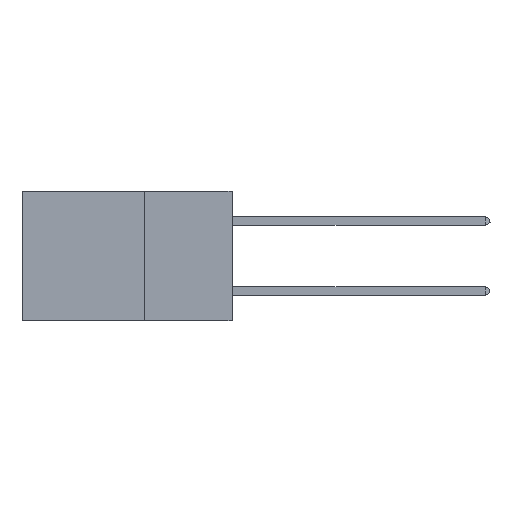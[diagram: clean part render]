
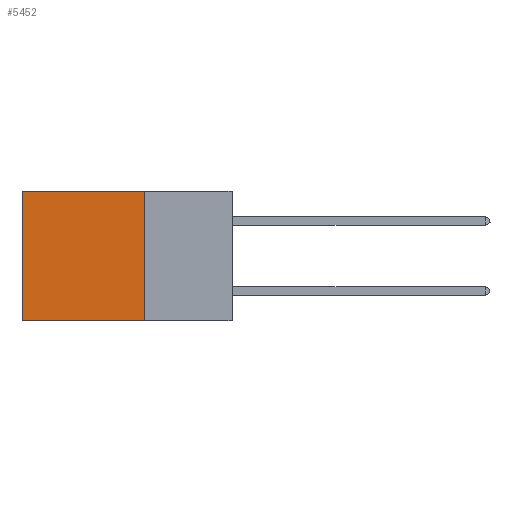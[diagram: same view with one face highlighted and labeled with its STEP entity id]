
A CAD part, left-side view. The second image highlights one B-rep face of the part: STEP entity #5452.
In plain terms, the highlighted planar face has unit normal (-1, 0, 0).
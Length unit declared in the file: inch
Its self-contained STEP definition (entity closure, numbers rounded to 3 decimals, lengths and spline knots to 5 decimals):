
#596 = VERTEX_POINT ( 'NONE', #9469 ) ;
#721 = EDGE_LOOP ( 'NONE', ( #8017, #20499, #3703, #16125 ) ) ;
#2265 = DIRECTION ( 'NONE',  ( 0., 1., 0. ) ) ;
#3703 = ORIENTED_EDGE ( 'NONE', *, *, #10382, .F. ) ;
#3742 = LINE ( 'NONE', #13536, #12031 ) ;
#3976 = CARTESIAN_POINT ( 'NONE',  ( 0.2875, 0.6, 0. ) ) ;
#4491 = VECTOR ( 'NONE', #18444, 39.37008 ) ;
#5256 = DIRECTION ( 'NONE',  ( 0., 1., 0. ) ) ;
#5452 = ADVANCED_FACE ( 'NONE', ( #7688 ), #12800, .F. ) ;
#6982 = EDGE_CURVE ( 'NONE', #16123, #16011, #18813, .T. ) ;
#7223 = VECTOR ( 'NONE', #9076, 39.37008 ) ;
#7688 = FACE_OUTER_BOUND ( 'NONE', #721, .T. ) ;
#8017 = ORIENTED_EDGE ( 'NONE', *, *, #8840, .T. ) ;
#8128 = VERTEX_POINT ( 'NONE', #19693 ) ;
#8840 = EDGE_CURVE ( 'NONE', #16011, #596, #12239, .T. ) ;
#9076 = DIRECTION ( 'NONE',  ( 0., 0., -1. ) ) ;
#9469 = CARTESIAN_POINT ( 'NONE',  ( 0.2875, 0.6, -0.37 ) ) ;
#10382 = EDGE_CURVE ( 'NONE', #16123, #8128, #18337, .T. ) ;
#11920 = CARTESIAN_POINT ( 'NONE',  ( 0.2875, 0.6, 0. ) ) ;
#12031 = VECTOR ( 'NONE', #5256, 39.37008 ) ;
#12239 = LINE ( 'NONE', #11920, #7223 ) ;
#12700 = DIRECTION ( 'NONE',  ( 1., 0., 0. ) ) ;
#12800 = PLANE ( 'NONE',  #15251 ) ;
#13358 = VECTOR ( 'NONE', #2265, 39.37008 ) ;
#13536 = CARTESIAN_POINT ( 'NONE',  ( 0.2875, 0.25, -0.37 ) ) ;
#14340 = CARTESIAN_POINT ( 'NONE',  ( 0.2875, 0.25, 0. ) ) ;
#15251 = AXIS2_PLACEMENT_3D ( 'NONE', #14340, #12700, #17719 ) ;
#16011 = VERTEX_POINT ( 'NONE', #3976 ) ;
#16123 = VERTEX_POINT ( 'NONE', #21270 ) ;
#16125 = ORIENTED_EDGE ( 'NONE', *, *, #6982, .T. ) ;
#17187 = CARTESIAN_POINT ( 'NONE',  ( 0.2875, 0.25, 0. ) ) ;
#17719 = DIRECTION ( 'NONE',  ( 0., 0., -1. ) ) ;
#18337 = LINE ( 'NONE', #19970, #4491 ) ;
#18444 = DIRECTION ( 'NONE',  ( 0., 0., -1. ) ) ;
#18813 = LINE ( 'NONE', #17187, #13358 ) ;
#19693 = CARTESIAN_POINT ( 'NONE',  ( 0.2875, 0.25, -0.37 ) ) ;
#19970 = CARTESIAN_POINT ( 'NONE',  ( 0.2875, 0.25, 0. ) ) ;
#20170 = EDGE_CURVE ( 'NONE', #8128, #596, #3742, .T. ) ;
#20499 = ORIENTED_EDGE ( 'NONE', *, *, #20170, .F. ) ;
#21270 = CARTESIAN_POINT ( 'NONE',  ( 0.2875, 0.25, 0. ) ) ;
